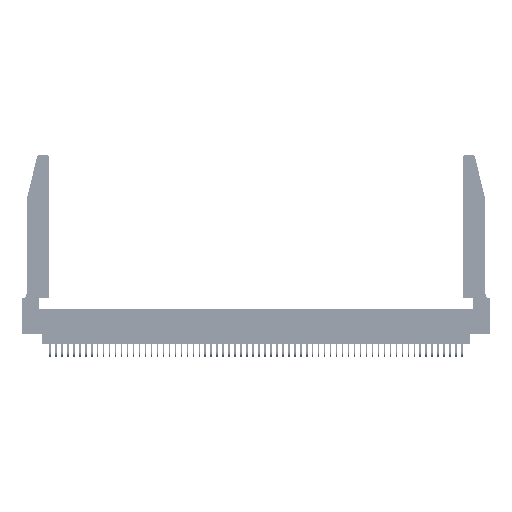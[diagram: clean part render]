
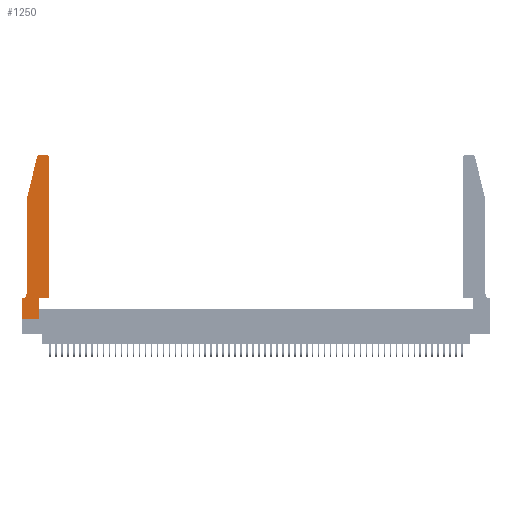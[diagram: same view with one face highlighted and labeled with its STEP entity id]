
A CAD part, top view. The second image highlights one B-rep face of the part: STEP entity #1250.
In plain terms, the highlighted planar face has unit normal (0, 0, 1).
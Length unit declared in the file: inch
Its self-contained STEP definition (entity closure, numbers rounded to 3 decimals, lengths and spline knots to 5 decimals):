
#1024 = VECTOR ( 'NONE', #54147, 39.37008 ) ;
#1250 = ADVANCED_FACE ( 'NONE', ( #6079 ), #20907, .T. ) ;
#1608 = EDGE_CURVE ( 'NONE', #32380, #46945, #54836, .T. ) ;
#1821 = VECTOR ( 'NONE', #29849, 39.37008 ) ;
#2134 = DIRECTION ( 'NONE',  ( 0., -1., 0. ) ) ;
#2323 = VERTEX_POINT ( 'NONE', #24482 ) ;
#2374 = LINE ( 'NONE', #45578, #10759 ) ;
#3146 = DIRECTION ( 'NONE',  ( 1., 0., 0. ) ) ;
#3205 = AXIS2_PLACEMENT_3D ( 'NONE', #16582, #39037, #12297 ) ;
#4309 = LINE ( 'NONE', #14140, #48938 ) ;
#4529 = DIRECTION ( 'NONE',  ( 0., -1., 0. ) ) ;
#6079 = FACE_OUTER_BOUND ( 'NONE', #19690, .T. ) ;
#6125 = EDGE_CURVE ( 'NONE', #20558, #41172, #18656, .T. ) ;
#6568 = DIRECTION ( 'NONE',  ( 1., 0., 0. ) ) ;
#7436 = CARTESIAN_POINT ( 'NONE',  ( 0.4505, 0.35, 0.37 ) ) ;
#7648 = DIRECTION ( 'NONE',  ( 1., 0., 0. ) ) ;
#7690 = ORIENTED_EDGE ( 'NONE', *, *, #25079, .T. ) ;
#8385 = VERTEX_POINT ( 'NONE', #30065 ) ;
#8526 = EDGE_CURVE ( 'NONE', #46945, #20558, #14247, .T. ) ;
#9103 = CARTESIAN_POINT ( 'NONE',  ( 0., 0.35, 0.37 ) ) ;
#9246 = ORIENTED_EDGE ( 'NONE', *, *, #29233, .T. ) ;
#9779 = VERTEX_POINT ( 'NONE', #13167 ) ;
#10390 = VERTEX_POINT ( 'NONE', #17379 ) ;
#10460 = EDGE_CURVE ( 'NONE', #41172, #48150, #50960, .T. ) ;
#10759 = VECTOR ( 'NONE', #18833, 39.37008 ) ;
#11407 = DIRECTION ( 'NONE',  ( 0., 0., 1. ) ) ;
#11722 = CARTESIAN_POINT ( 'NONE',  ( 0.0755, 2., 0.37 ) ) ;
#12297 = DIRECTION ( 'NONE',  ( -1., 0., 0. ) ) ;
#12664 = CARTESIAN_POINT ( 'NONE',  ( 0.2605, 2.75, 0.37 ) ) ;
#13167 = CARTESIAN_POINT ( 'NONE',  ( 0.2865, 0.35, 0.37 ) ) ;
#13537 = LINE ( 'NONE', #22412, #1024 ) ;
#14140 = CARTESIAN_POINT ( 'NONE',  ( 0.4505, 0.35, 0.37 ) ) ;
#14247 = CIRCLE ( 'NONE', #3205, 0.07 ) ;
#14330 = LINE ( 'NONE', #11722, #1821 ) ;
#15444 = ORIENTED_EDGE ( 'NONE', *, *, #10460, .T. ) ;
#16582 = CARTESIAN_POINT ( 'NONE',  ( 0.0055, 0.42, 0.37 ) ) ;
#17010 = ORIENTED_EDGE ( 'NONE', *, *, #8526, .T. ) ;
#17379 = CARTESIAN_POINT ( 'NONE',  ( 0.4205, 2.75, 0.37 ) ) ;
#17449 = ORIENTED_EDGE ( 'NONE', *, *, #30433, .T. ) ;
#18656 = LINE ( 'NONE', #45140, #28432 ) ;
#18833 = DIRECTION ( 'NONE',  ( 1., 0., 0. ) ) ;
#19690 = EDGE_LOOP ( 'NONE', ( #37243, #47432, #26211, #36331, #17010, #35877, #15444, #7690, #38405, #9246, #40079, #17449 ) ) ;
#20018 = LINE ( 'NONE', #7436, #54171 ) ;
#20162 = AXIS2_PLACEMENT_3D ( 'NONE', #50780, #55245, #28541 ) ;
#20200 = CARTESIAN_POINT ( 'NONE',  ( 0.284, 2.72, 0.37 ) ) ;
#20558 = VERTEX_POINT ( 'NONE', #23480 ) ;
#20907 = PLANE ( 'NONE',  #32470 ) ;
#22412 = CARTESIAN_POINT ( 'NONE',  ( 0.2865, 0.35, 0.37 ) ) ;
#23357 = VECTOR ( 'NONE', #35831, 39.37008 ) ;
#23480 = CARTESIAN_POINT ( 'NONE',  ( 0.0055, 0.35, 0.37 ) ) ;
#24482 = CARTESIAN_POINT ( 'NONE',  ( 0.284, 2.75, 0.37 ) ) ;
#25079 = EDGE_CURVE ( 'NONE', #48150, #45745, #2374, .T. ) ;
#25380 = DIRECTION ( 'NONE',  ( 0., 0., 1. ) ) ;
#26211 = ORIENTED_EDGE ( 'NONE', *, *, #42459, .T. ) ;
#26785 = DIRECTION ( 'NONE',  ( -1., 0., 0. ) ) ;
#28432 = VECTOR ( 'NONE', #26785, 39.37008 ) ;
#28541 = DIRECTION ( 'NONE',  ( 1., 0., 0. ) ) ;
#28623 = CARTESIAN_POINT ( 'NONE',  ( 0.25487, 2.72718, 0.37 ) ) ;
#28938 = LINE ( 'NONE', #12664, #23357 ) ;
#29233 = EDGE_CURVE ( 'NONE', #9779, #54057, #20018, .T. ) ;
#29849 = DIRECTION ( 'NONE',  ( -0.239, -0.971, 0. ) ) ;
#30065 = CARTESIAN_POINT ( 'NONE',  ( 0.4505, 2.72, 0.37 ) ) ;
#30433 = EDGE_CURVE ( 'NONE', #8385, #10390, #40814, .T. ) ;
#30852 = CARTESIAN_POINT ( 'NONE',  ( 0., 0., 0.37 ) ) ;
#31082 = VERTEX_POINT ( 'NONE', #28623 ) ;
#32380 = VERTEX_POINT ( 'NONE', #51908 ) ;
#32470 = AXIS2_PLACEMENT_3D ( 'NONE', #38661, #25380, #7648 ) ;
#32554 = CARTESIAN_POINT ( 'NONE',  ( 0.0755, 2., 0.37 ) ) ;
#33432 = EDGE_CURVE ( 'NONE', #10390, #2323, #28938, .T. ) ;
#33920 = VECTOR ( 'NONE', #2134, 39.37008 ) ;
#35831 = DIRECTION ( 'NONE',  ( -1., 0., 0. ) ) ;
#35877 = ORIENTED_EDGE ( 'NONE', *, *, #6125, .T. ) ;
#36331 = ORIENTED_EDGE ( 'NONE', *, *, #1608, .T. ) ;
#36400 = CARTESIAN_POINT ( 'NONE',  ( 0.2865, 0., 0.37 ) ) ;
#36594 = CARTESIAN_POINT ( 'NONE',  ( 0., 0., 0.37 ) ) ;
#36979 = DIRECTION ( 'NONE',  ( 0., 1., 0. ) ) ;
#37052 = VECTOR ( 'NONE', #4529, 39.37008 ) ;
#37222 = EDGE_CURVE ( 'NONE', #2323, #31082, #43857, .T. ) ;
#37243 = ORIENTED_EDGE ( 'NONE', *, *, #33432, .T. ) ;
#37581 = AXIS2_PLACEMENT_3D ( 'NONE', #20200, #11407, #6568 ) ;
#38405 = ORIENTED_EDGE ( 'NONE', *, *, #49587, .T. ) ;
#38661 = CARTESIAN_POINT ( 'NONE',  ( 0., 0.35, 0.37 ) ) ;
#38683 = CARTESIAN_POINT ( 'NONE',  ( 0.0755, 0.42, 0.37 ) ) ;
#39037 = DIRECTION ( 'NONE',  ( 0., 0., -1. ) ) ;
#40079 = ORIENTED_EDGE ( 'NONE', *, *, #45753, .T. ) ;
#40814 = CIRCLE ( 'NONE', #20162, 0.03 ) ;
#41172 = VERTEX_POINT ( 'NONE', #9103 ) ;
#42459 = EDGE_CURVE ( 'NONE', #31082, #32380, #14330, .T. ) ;
#43857 = CIRCLE ( 'NONE', #37581, 0.03 ) ;
#45140 = CARTESIAN_POINT ( 'NONE',  ( 0.0755, 0.35, 0.37 ) ) ;
#45578 = CARTESIAN_POINT ( 'NONE',  ( 0., 0., 0.37 ) ) ;
#45745 = VERTEX_POINT ( 'NONE', #36400 ) ;
#45753 = EDGE_CURVE ( 'NONE', #54057, #8385, #4309, .T. ) ;
#46945 = VERTEX_POINT ( 'NONE', #38683 ) ;
#47432 = ORIENTED_EDGE ( 'NONE', *, *, #37222, .T. ) ;
#48150 = VERTEX_POINT ( 'NONE', #36594 ) ;
#48938 = VECTOR ( 'NONE', #36979, 39.37008 ) ;
#49587 = EDGE_CURVE ( 'NONE', #45745, #9779, #13537, .T. ) ;
#50780 = CARTESIAN_POINT ( 'NONE',  ( 0.4205, 2.72, 0.37 ) ) ;
#50960 = LINE ( 'NONE', #30852, #37052 ) ;
#51908 = CARTESIAN_POINT ( 'NONE',  ( 0.0755, 2., 0.37 ) ) ;
#54057 = VERTEX_POINT ( 'NONE', #56589 ) ;
#54147 = DIRECTION ( 'NONE',  ( 0., 1., 0. ) ) ;
#54171 = VECTOR ( 'NONE', #3146, 39.37008 ) ;
#54836 = LINE ( 'NONE', #32554, #33920 ) ;
#55245 = DIRECTION ( 'NONE',  ( 0., 0., 1. ) ) ;
#56589 = CARTESIAN_POINT ( 'NONE',  ( 0.4505, 0.35, 0.37 ) ) ;
